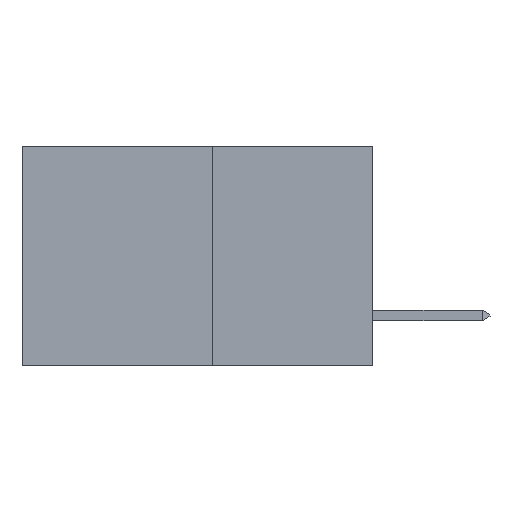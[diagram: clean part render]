
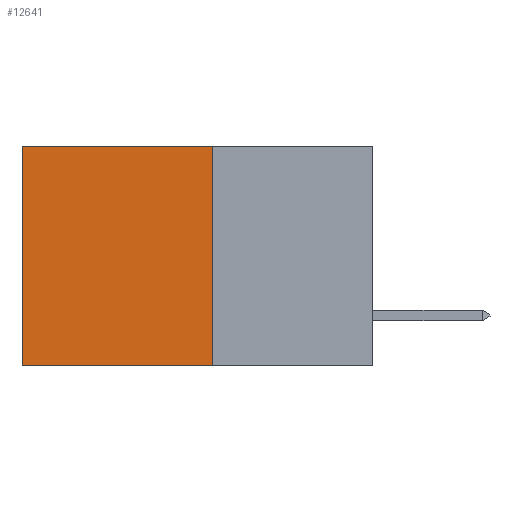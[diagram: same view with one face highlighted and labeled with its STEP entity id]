
A CAD part, left-side view. The second image highlights one B-rep face of the part: STEP entity #12641.
In plain terms, the highlighted planar face has unit normal (-1, 0, 0).
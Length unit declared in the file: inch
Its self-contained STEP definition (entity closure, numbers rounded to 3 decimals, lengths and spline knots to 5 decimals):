
#1 = ORIENTED_EDGE ( 'NONE', *, *, #12669, .T. ) ;
#139 = CARTESIAN_POINT ( 'NONE',  ( 0.277, 0.27, -0.37 ) ) ;
#1501 = CARTESIAN_POINT ( 'NONE',  ( 0.277, 0.27, -0.37 ) ) ;
#2431 = DIRECTION ( 'NONE',  ( 0., 1., 0. ) ) ;
#2988 = LINE ( 'NONE', #7481, #18033 ) ;
#3318 = EDGE_CURVE ( 'NONE', #8829, #7984, #17439, .T. ) ;
#3389 = CARTESIAN_POINT ( 'NONE',  ( 0.277, 0.27, 0. ) ) ;
#3410 = DIRECTION ( 'NONE',  ( 0., 1., 0. ) ) ;
#3650 = CARTESIAN_POINT ( 'NONE',  ( 0.277, 0.27, -0.37 ) ) ;
#3783 = EDGE_CURVE ( 'NONE', #9410, #8829, #9659, .T. ) ;
#4498 = PLANE ( 'NONE',  #9011 ) ;
#4632 = DIRECTION ( 'NONE',  ( 0., 0., -1. ) ) ;
#5719 = EDGE_CURVE ( 'NONE', #9410, #11927, #13116, .T. ) ;
#5772 = VECTOR ( 'NONE', #14447, 39.37008 ) ;
#5792 = VECTOR ( 'NONE', #2431, 39.37008 ) ;
#5963 = DIRECTION ( 'NONE',  ( 0., 0., -1. ) ) ;
#6633 = EDGE_LOOP ( 'NONE', ( #1, #13055, #12639, #12408 ) ) ;
#7481 = CARTESIAN_POINT ( 'NONE',  ( 0.277, 0.59, -0.37 ) ) ;
#7512 = CARTESIAN_POINT ( 'NONE',  ( 0.277, 0.59, 0. ) ) ;
#7984 = VERTEX_POINT ( 'NONE', #14411 ) ;
#8829 = VERTEX_POINT ( 'NONE', #139 ) ;
#9011 = AXIS2_PLACEMENT_3D ( 'NONE', #1501, #14711, #5963 ) ;
#9410 = VERTEX_POINT ( 'NONE', #16291 ) ;
#9659 = LINE ( 'NONE', #17241, #5772 ) ;
#11927 = VERTEX_POINT ( 'NONE', #7512 ) ;
#12408 = ORIENTED_EDGE ( 'NONE', *, *, #5719, .T. ) ;
#12639 = ORIENTED_EDGE ( 'NONE', *, *, #3783, .F. ) ;
#12641 = ADVANCED_FACE ( 'NONE', ( #15526 ), #4498, .F. ) ;
#12669 = EDGE_CURVE ( 'NONE', #11927, #7984, #2988, .T. ) ;
#13055 = ORIENTED_EDGE ( 'NONE', *, *, #3318, .F. ) ;
#13116 = LINE ( 'NONE', #3389, #16562 ) ;
#14411 = CARTESIAN_POINT ( 'NONE',  ( 0.277, 0.59, -0.37 ) ) ;
#14447 = DIRECTION ( 'NONE',  ( 0., 0., -1. ) ) ;
#14711 = DIRECTION ( 'NONE',  ( 1., 0., 0. ) ) ;
#15526 = FACE_OUTER_BOUND ( 'NONE', #6633, .T. ) ;
#16291 = CARTESIAN_POINT ( 'NONE',  ( 0.277, 0.27, 0. ) ) ;
#16562 = VECTOR ( 'NONE', #3410, 39.37008 ) ;
#17241 = CARTESIAN_POINT ( 'NONE',  ( 0.277, 0.27, -0.37 ) ) ;
#17439 = LINE ( 'NONE', #3650, #5792 ) ;
#18033 = VECTOR ( 'NONE', #4632, 39.37008 ) ;
